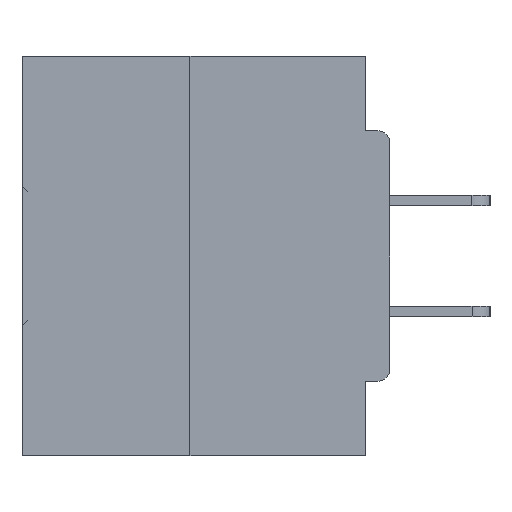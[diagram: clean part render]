
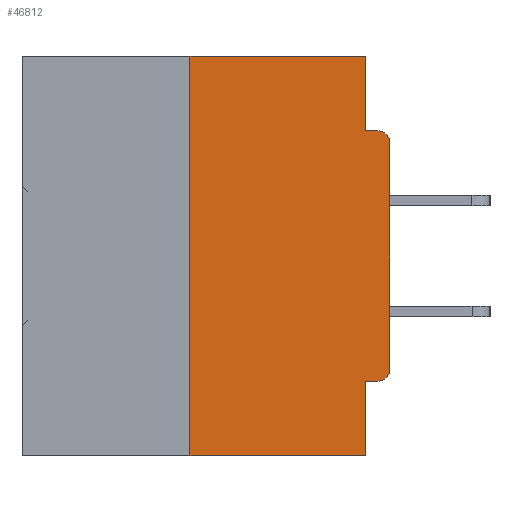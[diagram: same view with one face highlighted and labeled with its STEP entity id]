
A CAD part, left-side view. The second image highlights one B-rep face of the part: STEP entity #46812.
In plain terms, the highlighted planar face has unit normal (-1, 0, 0).
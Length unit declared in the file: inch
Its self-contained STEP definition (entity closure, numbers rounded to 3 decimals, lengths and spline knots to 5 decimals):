
#184 = CARTESIAN_POINT ( 'NONE',  ( 0., 0.015, -0.4065 ) ) ;
#556 = DIRECTION ( 'NONE',  ( 0., 0., 1. ) ) ;
#924 = CARTESIAN_POINT ( 'NONE',  ( 0., 0.031, -0.0935 ) ) ;
#1639 = FACE_OUTER_BOUND ( 'NONE', #37540, .T. ) ;
#2324 = ORIENTED_EDGE ( 'NONE', *, *, #29815, .F. ) ;
#3606 = DIRECTION ( 'NONE',  ( 0., 0., 1. ) ) ;
#3680 = VECTOR ( 'NONE', #19589, 39.37008 ) ;
#4645 = EDGE_CURVE ( 'NONE', #27829, #44810, #28095, .T. ) ;
#4753 = CARTESIAN_POINT ( 'NONE',  ( 0., 0., -0.3915 ) ) ;
#6197 = VECTOR ( 'NONE', #37927, 39.37008 ) ;
#6403 = VERTEX_POINT ( 'NONE', #30188 ) ;
#6890 = EDGE_CURVE ( 'NONE', #22949, #38132, #47330, .T. ) ;
#8502 = CARTESIAN_POINT ( 'NONE',  ( 0., 0.015, -0.3915 ) ) ;
#9267 = DIRECTION ( 'NONE',  ( 0., -1., 0. ) ) ;
#9863 = ORIENTED_EDGE ( 'NONE', *, *, #24055, .T. ) ;
#10334 = ORIENTED_EDGE ( 'NONE', *, *, #4645, .F. ) ;
#12302 = VECTOR ( 'NONE', #26692, 39.37008 ) ;
#13976 = LINE ( 'NONE', #41550, #3680 ) ;
#14507 = PLANE ( 'NONE',  #38708 ) ;
#14657 = DIRECTION ( 'NONE',  ( 0., -1., 0. ) ) ;
#14699 = AXIS2_PLACEMENT_3D ( 'NONE', #8502, #15878, #34201 ) ;
#15878 = DIRECTION ( 'NONE',  ( -1., 0., 0. ) ) ;
#15889 = ORIENTED_EDGE ( 'NONE', *, *, #18724, .F. ) ;
#16383 = CARTESIAN_POINT ( 'NONE',  ( 0., 0., -0.0935 ) ) ;
#16466 = CARTESIAN_POINT ( 'NONE',  ( 0., 0.031, 0. ) ) ;
#17346 = VECTOR ( 'NONE', #556, 39.37008 ) ;
#18494 = EDGE_CURVE ( 'NONE', #27396, #6403, #13976, .T. ) ;
#18724 = EDGE_CURVE ( 'NONE', #25810, #27396, #35867, .T. ) ;
#19589 = DIRECTION ( 'NONE',  ( 0., 0., -1. ) ) ;
#19811 = CIRCLE ( 'NONE', #14699, 0.015 ) ;
#19895 = VECTOR ( 'NONE', #3606, 39.37008 ) ;
#20385 = CARTESIAN_POINT ( 'NONE',  ( 0., 0.46, -0.5 ) ) ;
#20883 = CARTESIAN_POINT ( 'NONE',  ( 0., 0.25, -0.5 ) ) ;
#21278 = EDGE_CURVE ( 'NONE', #25810, #27796, #19811, .T. ) ;
#21836 = ORIENTED_EDGE ( 'NONE', *, *, #6890, .F. ) ;
#21940 = CARTESIAN_POINT ( 'NONE',  ( 0., 0.46, 0. ) ) ;
#22949 = VERTEX_POINT ( 'NONE', #34456 ) ;
#23522 = DIRECTION ( 'NONE',  ( 0., 0., -1. ) ) ;
#23960 = ORIENTED_EDGE ( 'NONE', *, *, #32678, .T. ) ;
#24055 = EDGE_CURVE ( 'NONE', #46217, #6403, #45045, .T. ) ;
#25592 = AXIS2_PLACEMENT_3D ( 'NONE', #28149, #31844, #35527 ) ;
#25810 = VERTEX_POINT ( 'NONE', #184 ) ;
#25833 = ORIENTED_EDGE ( 'NONE', *, *, #47285, .F. ) ;
#26692 = DIRECTION ( 'NONE',  ( 0., 1., 0. ) ) ;
#27396 = VERTEX_POINT ( 'NONE', #28929 ) ;
#27488 = LINE ( 'NONE', #40913, #34912 ) ;
#27796 = VERTEX_POINT ( 'NONE', #4753 ) ;
#27829 = VERTEX_POINT ( 'NONE', #924 ) ;
#28095 = LINE ( 'NONE', #16383, #6197 ) ;
#28149 = CARTESIAN_POINT ( 'NONE',  ( 0., 0.015, -0.1085 ) ) ;
#28712 = CARTESIAN_POINT ( 'NONE',  ( 0., 0.46, 0. ) ) ;
#28879 = EDGE_CURVE ( 'NONE', #42931, #44810, #32632, .T. ) ;
#28929 = CARTESIAN_POINT ( 'NONE',  ( 0., 0.031, -0.4065 ) ) ;
#29678 = LINE ( 'NONE', #45017, #19895 ) ;
#29815 = EDGE_CURVE ( 'NONE', #46217, #22949, #29678, .T. ) ;
#30188 = CARTESIAN_POINT ( 'NONE',  ( 0., 0.031, -0.5 ) ) ;
#30940 = ORIENTED_EDGE ( 'NONE', *, *, #18494, .F. ) ;
#30966 = CARTESIAN_POINT ( 'NONE',  ( 0., 0.015, -0.0935 ) ) ;
#31031 = CARTESIAN_POINT ( 'NONE',  ( 0., 0., -0.4065 ) ) ;
#31182 = LINE ( 'NONE', #44520, #17346 ) ;
#31844 = DIRECTION ( 'NONE',  ( -1., 0., 0. ) ) ;
#32632 = CIRCLE ( 'NONE', #25592, 0.015 ) ;
#32678 = EDGE_CURVE ( 'NONE', #27796, #42931, #31182, .T. ) ;
#34201 = DIRECTION ( 'NONE',  ( 0., 0., -1. ) ) ;
#34456 = CARTESIAN_POINT ( 'NONE',  ( 0., 0.25, 0. ) ) ;
#34912 = VECTOR ( 'NONE', #23522, 39.37008 ) ;
#35527 = DIRECTION ( 'NONE',  ( 0., 0., -1. ) ) ;
#35867 = LINE ( 'NONE', #31031, #12302 ) ;
#35926 = DIRECTION ( 'NONE',  ( 1., 0., 0. ) ) ;
#37540 = EDGE_LOOP ( 'NONE', ( #21836, #2324, #9863, #30940, #15889, #42565, #23960, #44665, #10334, #25833 ) ) ;
#37638 = VECTOR ( 'NONE', #14657, 39.37008 ) ;
#37927 = DIRECTION ( 'NONE',  ( 0., -1., 0. ) ) ;
#38132 = VERTEX_POINT ( 'NONE', #16466 ) ;
#38708 = AXIS2_PLACEMENT_3D ( 'NONE', #28712, #35926, #43249 ) ;
#39291 = VECTOR ( 'NONE', #9267, 39.37008 ) ;
#40913 = CARTESIAN_POINT ( 'NONE',  ( 0., 0.031, 0. ) ) ;
#41550 = CARTESIAN_POINT ( 'NONE',  ( 0., 0.031, -0.5 ) ) ;
#42565 = ORIENTED_EDGE ( 'NONE', *, *, #21278, .T. ) ;
#42931 = VERTEX_POINT ( 'NONE', #44487 ) ;
#43249 = DIRECTION ( 'NONE',  ( 0., 0., -1. ) ) ;
#44487 = CARTESIAN_POINT ( 'NONE',  ( 0., 0., -0.1085 ) ) ;
#44520 = CARTESIAN_POINT ( 'NONE',  ( 0., 0., 0. ) ) ;
#44665 = ORIENTED_EDGE ( 'NONE', *, *, #28879, .T. ) ;
#44810 = VERTEX_POINT ( 'NONE', #30966 ) ;
#45017 = CARTESIAN_POINT ( 'NONE',  ( 0., 0.25, 0. ) ) ;
#45045 = LINE ( 'NONE', #20385, #39291 ) ;
#46217 = VERTEX_POINT ( 'NONE', #20883 ) ;
#46812 = ADVANCED_FACE ( 'NONE', ( #1639 ), #14507, .F. ) ;
#47285 = EDGE_CURVE ( 'NONE', #38132, #27829, #27488, .T. ) ;
#47330 = LINE ( 'NONE', #21940, #37638 ) ;
